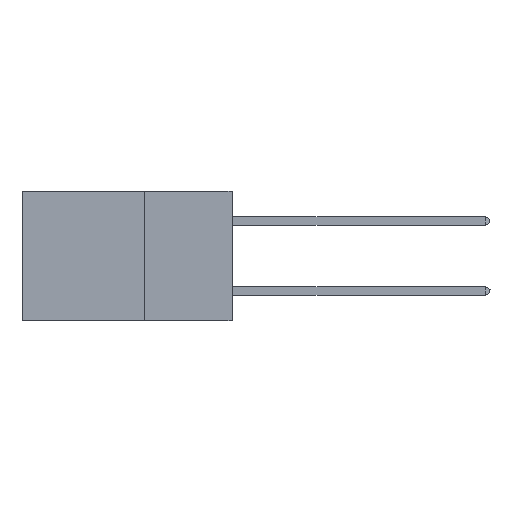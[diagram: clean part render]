
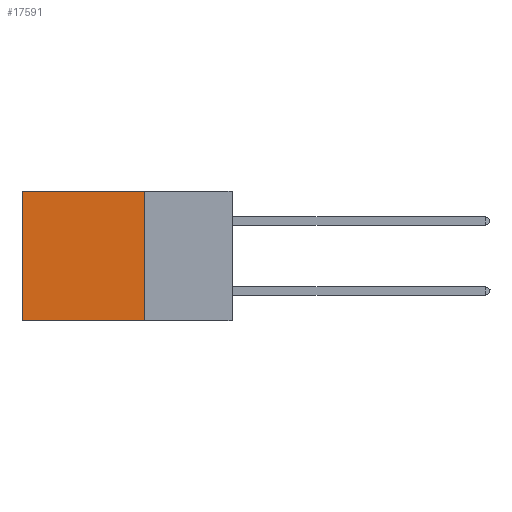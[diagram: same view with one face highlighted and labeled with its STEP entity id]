
A CAD part, left-side view. The second image highlights one B-rep face of the part: STEP entity #17591.
In plain terms, the highlighted planar face has unit normal (-1, 0, 0).
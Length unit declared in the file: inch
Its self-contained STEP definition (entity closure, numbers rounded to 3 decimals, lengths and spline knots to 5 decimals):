
#79 = DIRECTION ( 'NONE',  ( 1., 0., 0. ) ) ;
#144 = EDGE_CURVE ( 'NONE', #2665, #14282, #2390, .T. ) ;
#157 = EDGE_CURVE ( 'NONE', #22402, #14887, #10211, .T. ) ;
#1762 = CARTESIAN_POINT ( 'NONE',  ( 0.2875, 0.25, 0. ) ) ;
#2030 = LINE ( 'NONE', #13338, #7899 ) ;
#2092 = DIRECTION ( 'NONE',  ( 0., 1., 0. ) ) ;
#2390 = LINE ( 'NONE', #9605, #18070 ) ;
#2665 = VERTEX_POINT ( 'NONE', #13124 ) ;
#3789 = VECTOR ( 'NONE', #20002, 39.37008 ) ;
#5106 = ORIENTED_EDGE ( 'NONE', *, *, #20271, .T. ) ;
#7234 = FACE_OUTER_BOUND ( 'NONE', #15349, .T. ) ;
#7899 = VECTOR ( 'NONE', #9764, 39.37008 ) ;
#9605 = CARTESIAN_POINT ( 'NONE',  ( 0.2875, 0.25, 0. ) ) ;
#9764 = DIRECTION ( 'NONE',  ( 0., 0., -1. ) ) ;
#10211 = LINE ( 'NONE', #13113, #3789 ) ;
#10594 = PLANE ( 'NONE',  #23104 ) ;
#11710 = ORIENTED_EDGE ( 'NONE', *, *, #144, .T. ) ;
#12828 = CARTESIAN_POINT ( 'NONE',  ( 0.2875, 0.6, 0. ) ) ;
#13113 = CARTESIAN_POINT ( 'NONE',  ( 0.2875, 0.25, -0.37 ) ) ;
#13124 = CARTESIAN_POINT ( 'NONE',  ( 0.2875, 0.25, 0. ) ) ;
#13208 = DIRECTION ( 'NONE',  ( 0., 0., -1. ) ) ;
#13338 = CARTESIAN_POINT ( 'NONE',  ( 0.2875, 0.6, 0. ) ) ;
#14167 = ORIENTED_EDGE ( 'NONE', *, *, #15544, .F. ) ;
#14282 = VERTEX_POINT ( 'NONE', #12828 ) ;
#14887 = VERTEX_POINT ( 'NONE', #19393 ) ;
#15349 = EDGE_LOOP ( 'NONE', ( #5106, #17832, #14167, #11710 ) ) ;
#15544 = EDGE_CURVE ( 'NONE', #2665, #22402, #20994, .T. ) ;
#16226 = VECTOR ( 'NONE', #13208, 39.37008 ) ;
#17591 = ADVANCED_FACE ( 'NONE', ( #7234 ), #10594, .F. ) ;
#17832 = ORIENTED_EDGE ( 'NONE', *, *, #157, .F. ) ;
#18070 = VECTOR ( 'NONE', #2092, 39.37008 ) ;
#18694 = CARTESIAN_POINT ( 'NONE',  ( 0.2875, 0.25, 0. ) ) ;
#19393 = CARTESIAN_POINT ( 'NONE',  ( 0.2875, 0.6, -0.37 ) ) ;
#20002 = DIRECTION ( 'NONE',  ( 0., 1., 0. ) ) ;
#20271 = EDGE_CURVE ( 'NONE', #14282, #14887, #2030, .T. ) ;
#20994 = LINE ( 'NONE', #18694, #16226 ) ;
#21405 = DIRECTION ( 'NONE',  ( 0., 0., -1. ) ) ;
#22050 = CARTESIAN_POINT ( 'NONE',  ( 0.2875, 0.25, -0.37 ) ) ;
#22402 = VERTEX_POINT ( 'NONE', #22050 ) ;
#23104 = AXIS2_PLACEMENT_3D ( 'NONE', #1762, #79, #21405 ) ;
